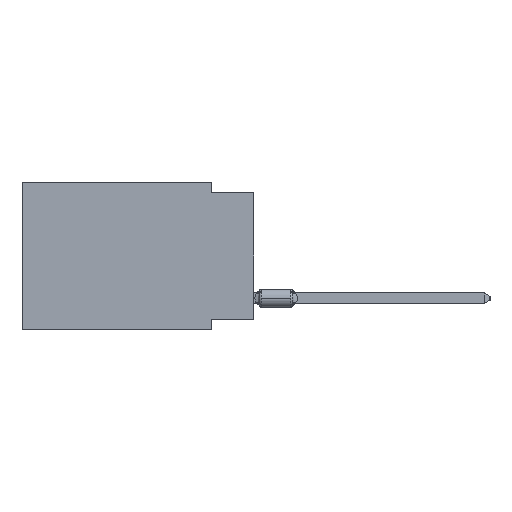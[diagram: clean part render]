
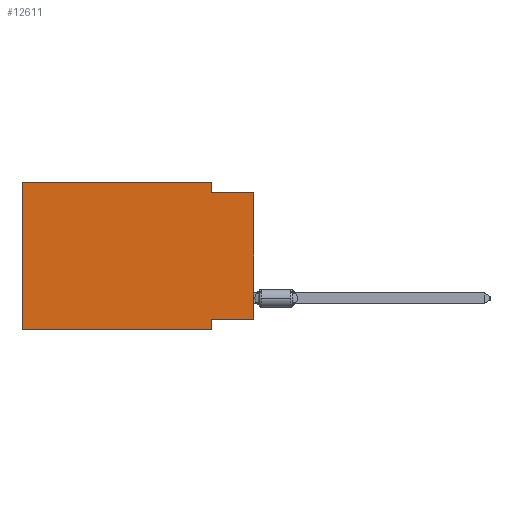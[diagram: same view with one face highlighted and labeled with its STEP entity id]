
A CAD part, left-side view. The second image highlights one B-rep face of the part: STEP entity #12611.
In plain terms, the highlighted planar face has unit normal (-1, 0, 0).
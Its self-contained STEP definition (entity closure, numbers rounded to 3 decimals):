
#650 = VERTEX_POINT ( 'NONE', #10834 ) ;
#884 = EDGE_CURVE ( 'NONE', #19319, #650, #6727, .T. ) ;
#2329 = ORIENTED_EDGE ( 'NONE', *, *, #10026, .T. ) ;
#2369 = CARTESIAN_POINT ( 'NONE',  ( 0., 13.97, 0. ) ) ;
#2779 = ORIENTED_EDGE ( 'NONE', *, *, #884, .T. ) ;
#2832 = VERTEX_POINT ( 'NONE', #8617 ) ;
#3127 = CARTESIAN_POINT ( 'NONE',  ( 0., 2.54, -8.255 ) ) ;
#4149 = DIRECTION ( 'NONE',  ( 0., -1., 0. ) ) ;
#4204 = LINE ( 'NONE', #33582, #6443 ) ;
#4396 = CARTESIAN_POINT ( 'NONE',  ( 0., 2.54, -8.89 ) ) ;
#5055 = ORIENTED_EDGE ( 'NONE', *, *, #34455, .F. ) ;
#5420 = VERTEX_POINT ( 'NONE', #35850 ) ;
#6443 = VECTOR ( 'NONE', #7117, 1000. ) ;
#6531 = DIRECTION ( 'NONE',  ( 1., 0., 0. ) ) ;
#6684 = DIRECTION ( 'NONE',  ( 0., 0., 1. ) ) ;
#6727 = LINE ( 'NONE', #14668, #13217 ) ;
#6818 = EDGE_CURVE ( 'NONE', #5420, #28438, #28823, .T. ) ;
#7117 = DIRECTION ( 'NONE',  ( 0., -1., 0. ) ) ;
#7359 = DIRECTION ( 'NONE',  ( 0., -1., 0. ) ) ;
#8584 = EDGE_CURVE ( 'NONE', #19319, #31185, #8861, .T. ) ;
#8617 = CARTESIAN_POINT ( 'NONE',  ( 0., 13.97, -8.89 ) ) ;
#8642 = CARTESIAN_POINT ( 'NONE',  ( 0., 0., -8.255 ) ) ;
#8643 = CARTESIAN_POINT ( 'NONE',  ( 0., 13.97, 0. ) ) ;
#8861 = LINE ( 'NONE', #26445, #24252 ) ;
#9263 = EDGE_LOOP ( 'NONE', ( #2779, #30840, #23230, #25311, #5055, #2329, #35940, #32751 ) ) ;
#10026 = EDGE_CURVE ( 'NONE', #2832, #33934, #4204, .T. ) ;
#10834 = CARTESIAN_POINT ( 'NONE',  ( 0., 0., -0.635 ) ) ;
#11058 = DIRECTION ( 'NONE',  ( 0., 0., 1. ) ) ;
#11382 = DIRECTION ( 'NONE',  ( 0., 1., 0. ) ) ;
#11813 = CARTESIAN_POINT ( 'NONE',  ( 0., 2.54, 0. ) ) ;
#12440 = VECTOR ( 'NONE', #4149, 1000. ) ;
#12611 = ADVANCED_FACE ( 'NONE', ( #17730 ), #32992, .F. ) ;
#13217 = VECTOR ( 'NONE', #6684, 1000. ) ;
#14668 = CARTESIAN_POINT ( 'NONE',  ( 0., 0., 0. ) ) ;
#15040 = EDGE_CURVE ( 'NONE', #17847, #5420, #21479, .T. ) ;
#15386 = DIRECTION ( 'NONE',  ( 0., 0., -1. ) ) ;
#17730 = FACE_OUTER_BOUND ( 'NONE', #9263, .T. ) ;
#17847 = VERTEX_POINT ( 'NONE', #32835 ) ;
#19319 = VERTEX_POINT ( 'NONE', #8642 ) ;
#19911 = VECTOR ( 'NONE', #22352, 1000. ) ;
#21479 = LINE ( 'NONE', #30165, #24058 ) ;
#21930 = CARTESIAN_POINT ( 'NONE',  ( 0., 0., -0.635 ) ) ;
#22352 = DIRECTION ( 'NONE',  ( 0., 0., -1. ) ) ;
#23230 = ORIENTED_EDGE ( 'NONE', *, *, #6818, .F. ) ;
#23494 = VECTOR ( 'NONE', #37901, 1000. ) ;
#24058 = VECTOR ( 'NONE', #7359, 1000. ) ;
#24252 = VECTOR ( 'NONE', #11382, 1000. ) ;
#25311 = ORIENTED_EDGE ( 'NONE', *, *, #15040, .F. ) ;
#26445 = CARTESIAN_POINT ( 'NONE',  ( 0., 0., -8.255 ) ) ;
#27698 = LINE ( 'NONE', #21930, #12440 ) ;
#28438 = VERTEX_POINT ( 'NONE', #38165 ) ;
#28823 = LINE ( 'NONE', #11813, #23494 ) ;
#30165 = CARTESIAN_POINT ( 'NONE',  ( 0., 13.97, 0. ) ) ;
#30840 = ORIENTED_EDGE ( 'NONE', *, *, #31551, .F. ) ;
#31150 = VECTOR ( 'NONE', #11058, 1000. ) ;
#31185 = VERTEX_POINT ( 'NONE', #3127 ) ;
#31417 = CARTESIAN_POINT ( 'NONE',  ( 0., 2.54, -8.89 ) ) ;
#31551 = EDGE_CURVE ( 'NONE', #28438, #650, #27698, .T. ) ;
#32751 = ORIENTED_EDGE ( 'NONE', *, *, #8584, .F. ) ;
#32835 = CARTESIAN_POINT ( 'NONE',  ( 0., 13.97, 0. ) ) ;
#32992 = PLANE ( 'NONE',  #34577 ) ;
#33582 = CARTESIAN_POINT ( 'NONE',  ( 0., 13.97, -8.89 ) ) ;
#33934 = VERTEX_POINT ( 'NONE', #4396 ) ;
#34455 = EDGE_CURVE ( 'NONE', #2832, #17847, #34825, .T. ) ;
#34577 = AXIS2_PLACEMENT_3D ( 'NONE', #8643, #6531, #15386 ) ;
#34825 = LINE ( 'NONE', #2369, #31150 ) ;
#35850 = CARTESIAN_POINT ( 'NONE',  ( 0., 2.54, 0. ) ) ;
#35940 = ORIENTED_EDGE ( 'NONE', *, *, #38103, .F. ) ;
#37221 = LINE ( 'NONE', #31417, #19911 ) ;
#37901 = DIRECTION ( 'NONE',  ( 0., 0., -1. ) ) ;
#38103 = EDGE_CURVE ( 'NONE', #31185, #33934, #37221, .T. ) ;
#38165 = CARTESIAN_POINT ( 'NONE',  ( 0., 2.54, -0.635 ) ) ;
